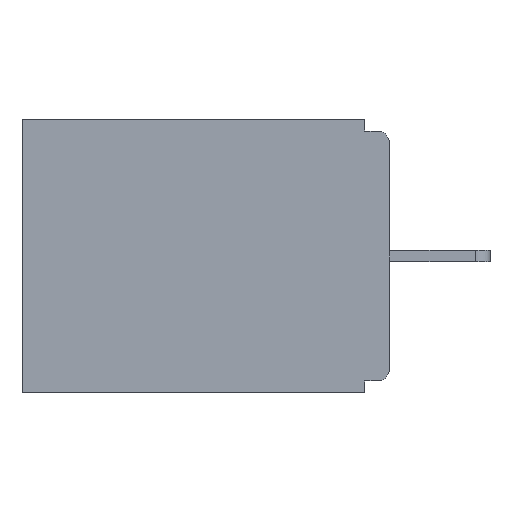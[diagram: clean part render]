
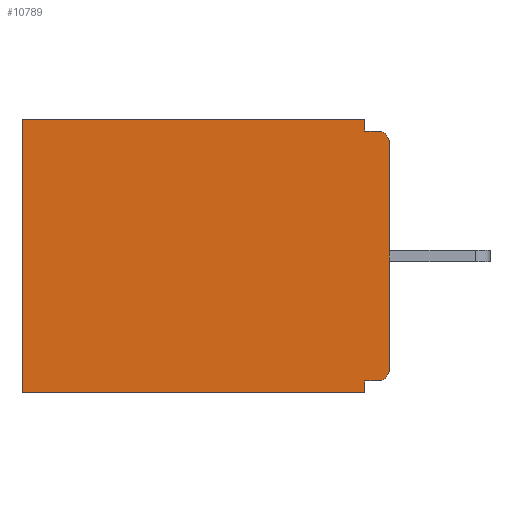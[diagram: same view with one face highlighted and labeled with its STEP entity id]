
A CAD part, left-side view. The second image highlights one B-rep face of the part: STEP entity #10789.
In plain terms, the highlighted planar face has unit normal (-1, 0, 0).
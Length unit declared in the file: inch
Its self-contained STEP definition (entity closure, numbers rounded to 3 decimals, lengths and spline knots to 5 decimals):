
#112 = CARTESIAN_POINT ( 'NONE',  ( 0.298, 0.015, -0.03 ) ) ;
#570 = DIRECTION ( 'NONE',  ( -1., 0., 0. ) ) ;
#905 = VECTOR ( 'NONE', #17451, 39.37008 ) ;
#1430 = LINE ( 'NONE', #8259, #9954 ) ;
#1438 = PLANE ( 'NONE',  #19822 ) ;
#1699 = LINE ( 'NONE', #14580, #10668 ) ;
#1769 = LINE ( 'NONE', #15499, #17035 ) ;
#2342 = CARTESIAN_POINT ( 'NONE',  ( 0.298, 0., 0. ) ) ;
#2489 = CARTESIAN_POINT ( 'NONE',  ( 0.298, 0., -0.03 ) ) ;
#2766 = AXIS2_PLACEMENT_3D ( 'NONE', #10200, #570, #11706 ) ;
#2968 = ORIENTED_EDGE ( 'NONE', *, *, #13498, .F. ) ;
#3263 = CARTESIAN_POINT ( 'NONE',  ( 0.298, 0.015, -0.015 ) ) ;
#3290 = EDGE_CURVE ( 'NONE', #11383, #13998, #1430, .T. ) ;
#3351 = EDGE_CURVE ( 'NONE', #19387, #13998, #16730, .T. ) ;
#3899 = CIRCLE ( 'NONE', #2766, 0.015 ) ;
#4001 = LINE ( 'NONE', #6074, #16013 ) ;
#4104 = EDGE_CURVE ( 'NONE', #18175, #14258, #15496, .T. ) ;
#4236 = EDGE_LOOP ( 'NONE', ( #14240, #6815, #14036, #12229, #16172, #16785, #9396, #2968, #18467, #14286 ) ) ;
#4708 = DIRECTION ( 'NONE',  ( -1., 0., 0. ) ) ;
#4719 = DIRECTION ( 'NONE',  ( 0., 0., -1. ) ) ;
#5207 = DIRECTION ( 'NONE',  ( 0., -1., 0. ) ) ;
#5813 = CARTESIAN_POINT ( 'NONE',  ( 0.298, 0.46, -0.343 ) ) ;
#6074 = CARTESIAN_POINT ( 'NONE',  ( 0.298, 0.031, -0.343 ) ) ;
#6650 = AXIS2_PLACEMENT_3D ( 'NONE', #112, #4708, #11304 ) ;
#6782 = DIRECTION ( 'NONE',  ( 0., 0., -1. ) ) ;
#6815 = ORIENTED_EDGE ( 'NONE', *, *, #10967, .F. ) ;
#7095 = CARTESIAN_POINT ( 'NONE',  ( 0.298, 0.031, -0.015 ) ) ;
#7222 = DIRECTION ( 'NONE',  ( 0., 0., -1. ) ) ;
#7343 = EDGE_CURVE ( 'NONE', #18175, #17782, #8594, .T. ) ;
#7583 = DIRECTION ( 'NONE',  ( 0., 1., 0. ) ) ;
#7667 = DIRECTION ( 'NONE',  ( 0., 0., -1. ) ) ;
#7683 = CARTESIAN_POINT ( 'NONE',  ( 0.298, 0.031, -0.343 ) ) ;
#7750 = DIRECTION ( 'NONE',  ( 0., 1., 0. ) ) ;
#7923 = EDGE_CURVE ( 'NONE', #19859, #19387, #14874, .T. ) ;
#8259 = CARTESIAN_POINT ( 'NONE',  ( 0.298, 0.46, 0. ) ) ;
#8594 = LINE ( 'NONE', #2342, #20356 ) ;
#9396 = ORIENTED_EDGE ( 'NONE', *, *, #7923, .F. ) ;
#9457 = FACE_OUTER_BOUND ( 'NONE', #4236, .T. ) ;
#9685 = CARTESIAN_POINT ( 'NONE',  ( 0.298, 0.031, 0. ) ) ;
#9954 = VECTOR ( 'NONE', #18071, 39.37008 ) ;
#10014 = CARTESIAN_POINT ( 'NONE',  ( 0.298, 0.031, -0.328 ) ) ;
#10092 = VECTOR ( 'NONE', #7750, 39.37008 ) ;
#10200 = CARTESIAN_POINT ( 'NONE',  ( 0.298, 0.015, -0.313 ) ) ;
#10668 = VECTOR ( 'NONE', #5207, 39.37008 ) ;
#10744 = VECTOR ( 'NONE', #7222, 39.37008 ) ;
#10789 = ADVANCED_FACE ( 'NONE', ( #9457 ), #1438, .F. ) ;
#10967 = EDGE_CURVE ( 'NONE', #19995, #14258, #1699, .T. ) ;
#11304 = DIRECTION ( 'NONE',  ( 0., 0., -1. ) ) ;
#11383 = VERTEX_POINT ( 'NONE', #20129 ) ;
#11706 = DIRECTION ( 'NONE',  ( 0., 0., -1. ) ) ;
#12229 = ORIENTED_EDGE ( 'NONE', *, *, #18336, .T. ) ;
#12384 = CARTESIAN_POINT ( 'NONE',  ( 0.298, 0., -0.328 ) ) ;
#12522 = CARTESIAN_POINT ( 'NONE',  ( 0.298, 0., 0. ) ) ;
#13192 = EDGE_CURVE ( 'NONE', #17189, #17782, #3899, .T. ) ;
#13498 = EDGE_CURVE ( 'NONE', #17189, #19859, #18274, .T. ) ;
#13628 = VERTEX_POINT ( 'NONE', #9685 ) ;
#13998 = VERTEX_POINT ( 'NONE', #5813 ) ;
#14036 = ORIENTED_EDGE ( 'NONE', *, *, #19564, .F. ) ;
#14096 = DIRECTION ( 'NONE',  ( 1., 0., 0. ) ) ;
#14240 = ORIENTED_EDGE ( 'NONE', *, *, #4104, .T. ) ;
#14258 = VERTEX_POINT ( 'NONE', #3263 ) ;
#14286 = ORIENTED_EDGE ( 'NONE', *, *, #7343, .F. ) ;
#14580 = CARTESIAN_POINT ( 'NONE',  ( 0.298, 0., -0.015 ) ) ;
#14874 = LINE ( 'NONE', #7683, #10744 ) ;
#15496 = CIRCLE ( 'NONE', #6650, 0.015 ) ;
#15499 = CARTESIAN_POINT ( 'NONE',  ( 0.298, 0., 0. ) ) ;
#16013 = VECTOR ( 'NONE', #7667, 39.37008 ) ;
#16172 = ORIENTED_EDGE ( 'NONE', *, *, #3290, .T. ) ;
#16730 = LINE ( 'NONE', #19108, #905 ) ;
#16785 = ORIENTED_EDGE ( 'NONE', *, *, #3351, .F. ) ;
#17035 = VECTOR ( 'NONE', #7583, 39.37008 ) ;
#17189 = VERTEX_POINT ( 'NONE', #18757 ) ;
#17451 = DIRECTION ( 'NONE',  ( 0., 1., 0. ) ) ;
#17782 = VERTEX_POINT ( 'NONE', #20241 ) ;
#18066 = CARTESIAN_POINT ( 'NONE',  ( 0.298, 0.031, -0.343 ) ) ;
#18071 = DIRECTION ( 'NONE',  ( 0., 0., -1. ) ) ;
#18175 = VERTEX_POINT ( 'NONE', #2489 ) ;
#18274 = LINE ( 'NONE', #12384, #10092 ) ;
#18336 = EDGE_CURVE ( 'NONE', #13628, #11383, #1769, .T. ) ;
#18467 = ORIENTED_EDGE ( 'NONE', *, *, #13192, .T. ) ;
#18757 = CARTESIAN_POINT ( 'NONE',  ( 0.298, 0.015, -0.328 ) ) ;
#19108 = CARTESIAN_POINT ( 'NONE',  ( 0.298, 0., -0.343 ) ) ;
#19387 = VERTEX_POINT ( 'NONE', #18066 ) ;
#19564 = EDGE_CURVE ( 'NONE', #13628, #19995, #4001, .T. ) ;
#19822 = AXIS2_PLACEMENT_3D ( 'NONE', #12522, #14096, #4719 ) ;
#19859 = VERTEX_POINT ( 'NONE', #10014 ) ;
#19995 = VERTEX_POINT ( 'NONE', #7095 ) ;
#20129 = CARTESIAN_POINT ( 'NONE',  ( 0.298, 0.46, 0. ) ) ;
#20241 = CARTESIAN_POINT ( 'NONE',  ( 0.298, 0., -0.313 ) ) ;
#20356 = VECTOR ( 'NONE', #6782, 39.37008 ) ;
